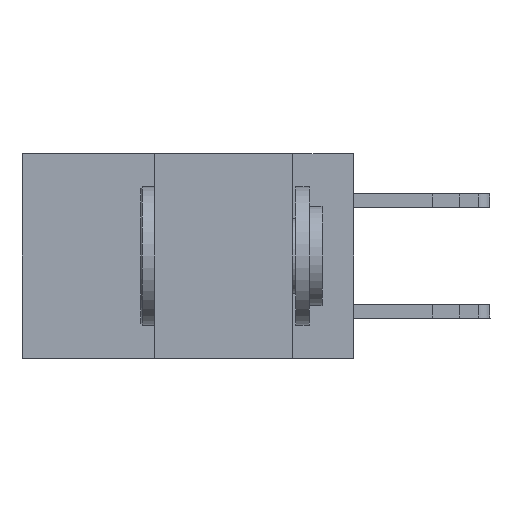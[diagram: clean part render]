
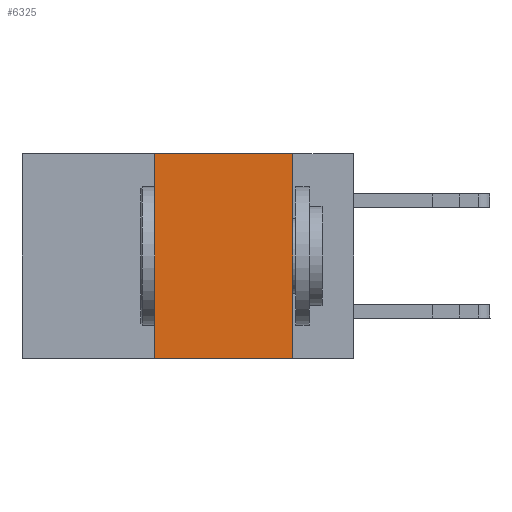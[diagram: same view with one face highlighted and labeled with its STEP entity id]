
A CAD part, left-side view. The second image highlights one B-rep face of the part: STEP entity #6325.
In plain terms, the highlighted planar face has unit normal (-1, 0, 0).
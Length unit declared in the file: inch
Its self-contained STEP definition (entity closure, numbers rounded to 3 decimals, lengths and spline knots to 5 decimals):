
#3004 = VERTEX_POINT ( 'NONE', #36150 ) ;
#4008 = EDGE_CURVE ( 'NONE', #3004, #19278, #7589, .T. ) ;
#4927 = CARTESIAN_POINT ( 'NONE',  ( 0., 0.11, 0. ) ) ;
#5979 = LINE ( 'NONE', #13275, #36932 ) ;
#6325 = ADVANCED_FACE ( 'NONE', ( #32699 ), #13545, .F. ) ;
#6542 = VERTEX_POINT ( 'NONE', #20122 ) ;
#7589 = LINE ( 'NONE', #22445, #22090 ) ;
#7593 = EDGE_LOOP ( 'NONE', ( #22542, #21823, #15446, #24118 ) ) ;
#9001 = CARTESIAN_POINT ( 'NONE',  ( 0., 0.6, -0.37 ) ) ;
#9658 = VERTEX_POINT ( 'NONE', #31559 ) ;
#13275 = CARTESIAN_POINT ( 'NONE',  ( 0., 0.36, 0. ) ) ;
#13545 = PLANE ( 'NONE',  #15825 ) ;
#14865 = VECTOR ( 'NONE', #31411, 39.37008 ) ;
#15446 = ORIENTED_EDGE ( 'NONE', *, *, #22363, .F. ) ;
#15825 = AXIS2_PLACEMENT_3D ( 'NONE', #34532, #16715, #37897 ) ;
#16199 = EDGE_CURVE ( 'NONE', #19278, #6542, #34081, .T. ) ;
#16715 = DIRECTION ( 'NONE',  ( 1., 0., 0. ) ) ;
#19278 = VERTEX_POINT ( 'NONE', #28922 ) ;
#20122 = CARTESIAN_POINT ( 'NONE',  ( 0., 0.11, -0.37 ) ) ;
#20238 = DIRECTION ( 'NONE',  ( 0., -1., 0. ) ) ;
#20842 = EDGE_CURVE ( 'NONE', #9658, #6542, #34160, .T. ) ;
#21823 = ORIENTED_EDGE ( 'NONE', *, *, #4008, .F. ) ;
#22090 = VECTOR ( 'NONE', #20238, 39.37008 ) ;
#22190 = DIRECTION ( 'NONE',  ( 0., 0., 1. ) ) ;
#22363 = EDGE_CURVE ( 'NONE', #9658, #3004, #5979, .T. ) ;
#22445 = CARTESIAN_POINT ( 'NONE',  ( 0., 0.6, 0. ) ) ;
#22542 = ORIENTED_EDGE ( 'NONE', *, *, #16199, .F. ) ;
#24118 = ORIENTED_EDGE ( 'NONE', *, *, #20842, .T. ) ;
#27210 = DIRECTION ( 'NONE',  ( 0., -1., 0. ) ) ;
#28922 = CARTESIAN_POINT ( 'NONE',  ( 0., 0.11, 0. ) ) ;
#31411 = DIRECTION ( 'NONE',  ( 0., 0., -1. ) ) ;
#31559 = CARTESIAN_POINT ( 'NONE',  ( 0., 0.36, -0.37 ) ) ;
#32699 = FACE_OUTER_BOUND ( 'NONE', #7593, .T. ) ;
#33209 = VECTOR ( 'NONE', #27210, 39.37008 ) ;
#34081 = LINE ( 'NONE', #4927, #14865 ) ;
#34160 = LINE ( 'NONE', #9001, #33209 ) ;
#34532 = CARTESIAN_POINT ( 'NONE',  ( 0., 0.6, 0. ) ) ;
#36150 = CARTESIAN_POINT ( 'NONE',  ( 0., 0.36, 0. ) ) ;
#36932 = VECTOR ( 'NONE', #22190, 39.37008 ) ;
#37897 = DIRECTION ( 'NONE',  ( 0., 0., -1. ) ) ;
